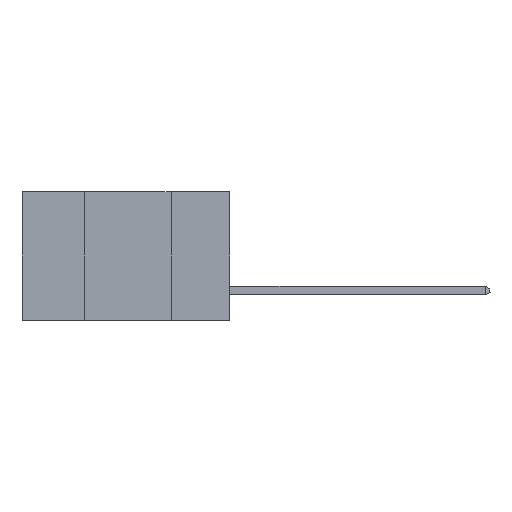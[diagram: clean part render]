
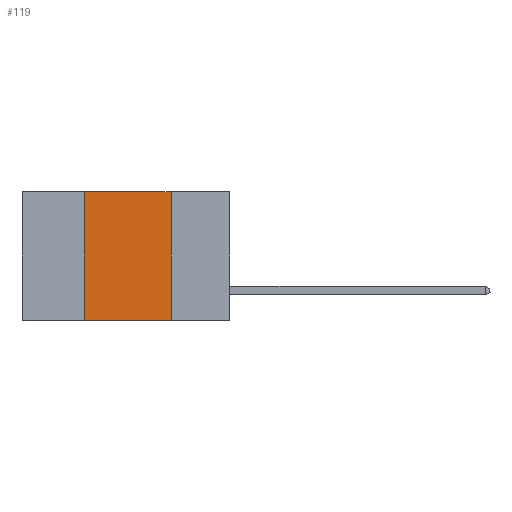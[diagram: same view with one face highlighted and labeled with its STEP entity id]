
A CAD part, left-side view. The second image highlights one B-rep face of the part: STEP entity #119.
In plain terms, the highlighted planar face has unit normal (-1, 0, 0).
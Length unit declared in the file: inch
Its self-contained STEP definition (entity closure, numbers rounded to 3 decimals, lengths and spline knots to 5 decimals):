
#119 = ADVANCED_FACE ( 'NONE', ( #5733 ), #1925, .F. ) ;
#317 = VECTOR ( 'NONE', #21820, 39.37008 ) ;
#572 = VERTEX_POINT ( 'NONE', #24843 ) ;
#1564 = LINE ( 'NONE', #6014, #317 ) ;
#1683 = DIRECTION ( 'NONE',  ( 1., 0., 0. ) ) ;
#1925 = PLANE ( 'NONE',  #14913 ) ;
#2236 = LINE ( 'NONE', #16781, #14987 ) ;
#2493 = EDGE_CURVE ( 'NONE', #22503, #15425, #22896, .T. ) ;
#3799 = CARTESIAN_POINT ( 'NONE',  ( 0., 0.17, -0.37 ) ) ;
#4901 = DIRECTION ( 'NONE',  ( 0., -1., 0. ) ) ;
#5690 = CARTESIAN_POINT ( 'NONE',  ( 0., 0.6, 0. ) ) ;
#5733 = FACE_OUTER_BOUND ( 'NONE', #7633, .T. ) ;
#6014 = CARTESIAN_POINT ( 'NONE',  ( 0., 0.17, 0. ) ) ;
#6212 = ORIENTED_EDGE ( 'NONE', *, *, #8289, .F. ) ;
#7584 = CARTESIAN_POINT ( 'NONE',  ( 0., 0.6, -0.37 ) ) ;
#7633 = EDGE_LOOP ( 'NONE', ( #6212, #19248, #11903, #14477 ) ) ;
#7666 = DIRECTION ( 'NONE',  ( 0., -1., 0. ) ) ;
#8289 = EDGE_CURVE ( 'NONE', #14697, #15425, #1564, .T. ) ;
#10471 = EDGE_CURVE ( 'NONE', #22503, #572, #12155, .T. ) ;
#10759 = CARTESIAN_POINT ( 'NONE',  ( 0., 0.42, -0.37 ) ) ;
#11903 = ORIENTED_EDGE ( 'NONE', *, *, #10471, .F. ) ;
#12155 = LINE ( 'NONE', #17991, #20728 ) ;
#14477 = ORIENTED_EDGE ( 'NONE', *, *, #2493, .T. ) ;
#14697 = VERTEX_POINT ( 'NONE', #25201 ) ;
#14913 = AXIS2_PLACEMENT_3D ( 'NONE', #5690, #1683, #23479 ) ;
#14987 = VECTOR ( 'NONE', #4901, 39.37008 ) ;
#15425 = VERTEX_POINT ( 'NONE', #3799 ) ;
#15680 = EDGE_CURVE ( 'NONE', #572, #14697, #2236, .T. ) ;
#16781 = CARTESIAN_POINT ( 'NONE',  ( 0., 0.6, 0. ) ) ;
#17991 = CARTESIAN_POINT ( 'NONE',  ( 0., 0.42, 0. ) ) ;
#19248 = ORIENTED_EDGE ( 'NONE', *, *, #15680, .F. ) ;
#20728 = VECTOR ( 'NONE', #25565, 39.37008 ) ;
#21820 = DIRECTION ( 'NONE',  ( 0., 0., -1. ) ) ;
#22503 = VERTEX_POINT ( 'NONE', #10759 ) ;
#22896 = LINE ( 'NONE', #7584, #24740 ) ;
#23479 = DIRECTION ( 'NONE',  ( 0., 0., -1. ) ) ;
#24740 = VECTOR ( 'NONE', #7666, 39.37008 ) ;
#24843 = CARTESIAN_POINT ( 'NONE',  ( 0., 0.42, 0. ) ) ;
#25201 = CARTESIAN_POINT ( 'NONE',  ( 0., 0.17, 0. ) ) ;
#25565 = DIRECTION ( 'NONE',  ( 0., 0., 1. ) ) ;
